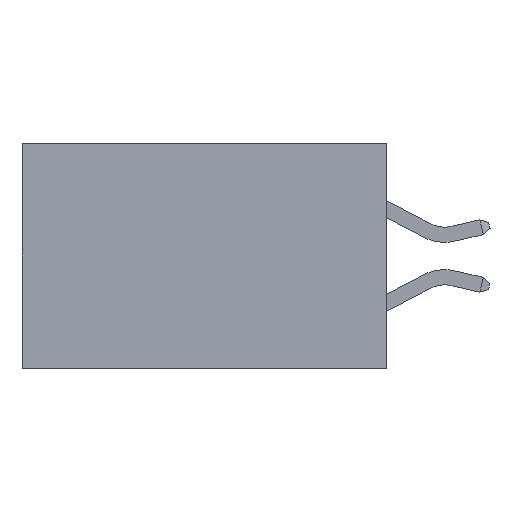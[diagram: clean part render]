
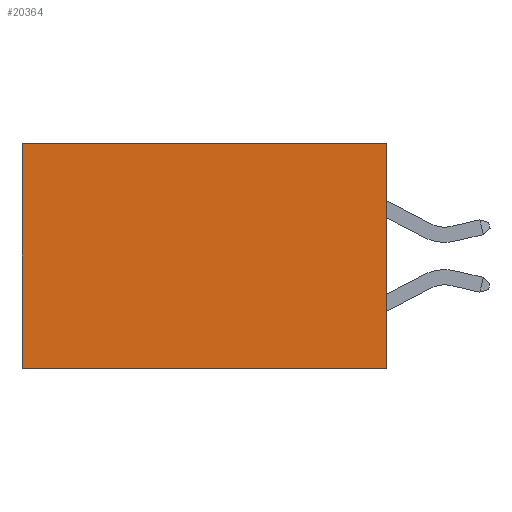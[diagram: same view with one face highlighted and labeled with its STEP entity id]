
A CAD part, left-side view. The second image highlights one B-rep face of the part: STEP entity #20364.
In plain terms, the highlighted planar face has unit normal (-1, 0, 0).
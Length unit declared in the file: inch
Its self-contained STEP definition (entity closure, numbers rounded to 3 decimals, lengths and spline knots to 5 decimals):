
#454 = CARTESIAN_POINT ( 'NONE',  ( 0.298, 0.6, 0. ) ) ;
#1077 = DIRECTION ( 'NONE',  ( 0., 0., -1. ) ) ;
#1736 = ORIENTED_EDGE ( 'NONE', *, *, #9662, .T. ) ;
#1943 = DIRECTION ( 'NONE',  ( 0., 1., 0. ) ) ;
#2198 = CARTESIAN_POINT ( 'NONE',  ( 0.298, 0., -0.37 ) ) ;
#2202 = VERTEX_POINT ( 'NONE', #8175 ) ;
#3069 = EDGE_LOOP ( 'NONE', ( #11781, #7306, #19303, #1736 ) ) ;
#3080 = EDGE_CURVE ( 'NONE', #16398, #2202, #12770, .T. ) ;
#3088 = CARTESIAN_POINT ( 'NONE',  ( 0.298, 0.6, 0. ) ) ;
#3395 = EDGE_CURVE ( 'NONE', #2202, #13214, #20210, .T. ) ;
#4412 = CARTESIAN_POINT ( 'NONE',  ( 0.298, 0., 0. ) ) ;
#4550 = CARTESIAN_POINT ( 'NONE',  ( 0.298, 0., 0. ) ) ;
#7306 = ORIENTED_EDGE ( 'NONE', *, *, #3395, .F. ) ;
#8175 = CARTESIAN_POINT ( 'NONE',  ( 0.298, 0., -0.37 ) ) ;
#8716 = VERTEX_POINT ( 'NONE', #454 ) ;
#8738 = CARTESIAN_POINT ( 'NONE',  ( 0.298, 0.6, -0.37 ) ) ;
#8808 = CARTESIAN_POINT ( 'NONE',  ( 0.298, 0., 0. ) ) ;
#9428 = LINE ( 'NONE', #4412, #17733 ) ;
#9662 = EDGE_CURVE ( 'NONE', #16398, #8716, #9428, .T. ) ;
#11376 = VECTOR ( 'NONE', #1943, 39.37008 ) ;
#11691 = DIRECTION ( 'NONE',  ( 1., 0., 0. ) ) ;
#11781 = ORIENTED_EDGE ( 'NONE', *, *, #22822, .T. ) ;
#11795 = CARTESIAN_POINT ( 'NONE',  ( 0.298, 0., 0. ) ) ;
#11921 = DIRECTION ( 'NONE',  ( 0., 0., -1. ) ) ;
#12770 = LINE ( 'NONE', #11795, #13323 ) ;
#13214 = VERTEX_POINT ( 'NONE', #8738 ) ;
#13323 = VECTOR ( 'NONE', #11921, 39.37008 ) ;
#14834 = FACE_OUTER_BOUND ( 'NONE', #3069, .T. ) ;
#16398 = VERTEX_POINT ( 'NONE', #8808 ) ;
#17217 = VECTOR ( 'NONE', #17265, 39.37008 ) ;
#17265 = DIRECTION ( 'NONE',  ( 0., 0., -1. ) ) ;
#17733 = VECTOR ( 'NONE', #22107, 39.37008 ) ;
#19303 = ORIENTED_EDGE ( 'NONE', *, *, #3080, .F. ) ;
#20210 = LINE ( 'NONE', #2198, #11376 ) ;
#20364 = ADVANCED_FACE ( 'NONE', ( #14834 ), #22232, .F. ) ;
#21118 = AXIS2_PLACEMENT_3D ( 'NONE', #4550, #11691, #1077 ) ;
#22107 = DIRECTION ( 'NONE',  ( 0., 1., 0. ) ) ;
#22232 = PLANE ( 'NONE',  #21118 ) ;
#22437 = LINE ( 'NONE', #3088, #17217 ) ;
#22822 = EDGE_CURVE ( 'NONE', #8716, #13214, #22437, .T. ) ;
